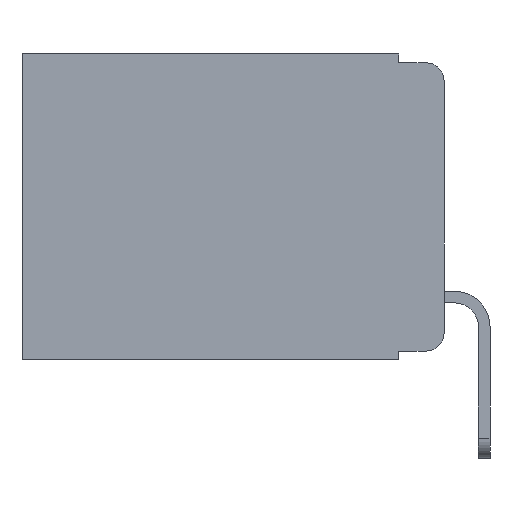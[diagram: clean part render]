
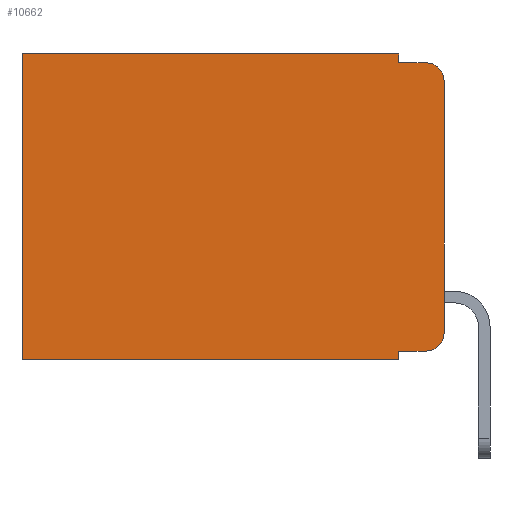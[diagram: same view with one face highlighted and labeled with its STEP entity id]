
A CAD part, left-side view. The second image highlights one B-rep face of the part: STEP entity #10662.
In plain terms, the highlighted planar face has unit normal (-1, 0, 0).
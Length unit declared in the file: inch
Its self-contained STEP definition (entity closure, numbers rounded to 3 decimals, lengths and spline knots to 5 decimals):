
#500 = FACE_OUTER_BOUND ( 'NONE', #8972, .T. ) ;
#1177 = CARTESIAN_POINT ( 'NONE',  ( 0.298, 0.051, 0. ) ) ;
#1775 = CARTESIAN_POINT ( 'NONE',  ( 0.298, 0.473, 0. ) ) ;
#1966 = VECTOR ( 'NONE', #8646, 39.37008 ) ;
#2136 = AXIS2_PLACEMENT_3D ( 'NONE', #11107, #2188, #13180 ) ;
#2175 = LINE ( 'NONE', #10441, #15450 ) ;
#2188 = DIRECTION ( 'NONE',  ( -1., 0., 0. ) ) ;
#2218 = ORIENTED_EDGE ( 'NONE', *, *, #2560, .F. ) ;
#2294 = EDGE_CURVE ( 'NONE', #3955, #2691, #2865, .T. ) ;
#2340 = VECTOR ( 'NONE', #8804, 39.37008 ) ;
#2560 = EDGE_CURVE ( 'NONE', #14445, #5333, #2175, .T. ) ;
#2691 = VERTEX_POINT ( 'NONE', #1775 ) ;
#2821 = CARTESIAN_POINT ( 'NONE',  ( 0.298, 0., 0. ) ) ;
#2848 = DIRECTION ( 'NONE',  ( 0., 1., 0. ) ) ;
#2865 = LINE ( 'NONE', #5798, #1966 ) ;
#2953 = VERTEX_POINT ( 'NONE', #11957 ) ;
#3133 = ORIENTED_EDGE ( 'NONE', *, *, #11868, .F. ) ;
#3510 = VERTEX_POINT ( 'NONE', #8682 ) ;
#3591 = ORIENTED_EDGE ( 'NONE', *, *, #7994, .T. ) ;
#3955 = VERTEX_POINT ( 'NONE', #4451 ) ;
#4451 = CARTESIAN_POINT ( 'NONE',  ( 0.298, 0.051, 0. ) ) ;
#5227 = ORIENTED_EDGE ( 'NONE', *, *, #6734, .T. ) ;
#5333 = VERTEX_POINT ( 'NONE', #7651 ) ;
#5467 = ORIENTED_EDGE ( 'NONE', *, *, #2294, .T. ) ;
#5698 = CARTESIAN_POINT ( 'NONE',  ( 0.298, 0.473, 0. ) ) ;
#5716 = CARTESIAN_POINT ( 'NONE',  ( 0.298, 0.051, -0.343 ) ) ;
#5798 = CARTESIAN_POINT ( 'NONE',  ( 0.298, 0., 0. ) ) ;
#5954 = VERTEX_POINT ( 'NONE', #15307 ) ;
#6241 = LINE ( 'NONE', #5698, #2340 ) ;
#6310 = CARTESIAN_POINT ( 'NONE',  ( 0.298, 0., -0.03 ) ) ;
#6734 = EDGE_CURVE ( 'NONE', #14445, #11534, #11903, .T. ) ;
#6886 = VECTOR ( 'NONE', #10620, 39.37008 ) ;
#6890 = VERTEX_POINT ( 'NONE', #8103 ) ;
#7211 = DIRECTION ( 'NONE',  ( 0., 0., -1. ) ) ;
#7340 = EDGE_CURVE ( 'NONE', #6890, #11534, #14330, .T. ) ;
#7443 = ORIENTED_EDGE ( 'NONE', *, *, #7914, .F. ) ;
#7535 = EDGE_CURVE ( 'NONE', #3955, #6890, #14315, .T. ) ;
#7651 = CARTESIAN_POINT ( 'NONE',  ( 0.298, 0., -0.313 ) ) ;
#7773 = VERTEX_POINT ( 'NONE', #5716 ) ;
#7779 = EDGE_CURVE ( 'NONE', #2691, #5954, #6241, .T. ) ;
#7889 = VECTOR ( 'NONE', #16439, 39.37008 ) ;
#7914 = EDGE_CURVE ( 'NONE', #2953, #7773, #16434, .T. ) ;
#7994 = EDGE_CURVE ( 'NONE', #2953, #3510, #12481, .T. ) ;
#8088 = ORIENTED_EDGE ( 'NONE', *, *, #7340, .F. ) ;
#8102 = ORIENTED_EDGE ( 'NONE', *, *, #8116, .T. ) ;
#8103 = CARTESIAN_POINT ( 'NONE',  ( 0.298, 0.051, -0.01 ) ) ;
#8116 = EDGE_CURVE ( 'NONE', #3510, #5333, #12986, .T. ) ;
#8257 = VECTOR ( 'NONE', #2848, 39.37008 ) ;
#8520 = PLANE ( 'NONE',  #10158 ) ;
#8646 = DIRECTION ( 'NONE',  ( 0., 1., 0. ) ) ;
#8682 = CARTESIAN_POINT ( 'NONE',  ( 0.298, 0.02, -0.333 ) ) ;
#8804 = DIRECTION ( 'NONE',  ( 0., 0., -1. ) ) ;
#8972 = EDGE_LOOP ( 'NONE', ( #2218, #5227, #8088, #15824, #5467, #9133, #3133, #7443, #3591, #8102 ) ) ;
#9133 = ORIENTED_EDGE ( 'NONE', *, *, #7779, .T. ) ;
#10158 = AXIS2_PLACEMENT_3D ( 'NONE', #2821, #14542, #7211 ) ;
#10441 = CARTESIAN_POINT ( 'NONE',  ( 0.298, 0., 0. ) ) ;
#10450 = DIRECTION ( 'NONE',  ( 0., -1., 0. ) ) ;
#10620 = DIRECTION ( 'NONE',  ( 0., 0., -1. ) ) ;
#10647 = AXIS2_PLACEMENT_3D ( 'NONE', #13116, #11872, #11854 ) ;
#10662 = ADVANCED_FACE ( 'NONE', ( #500 ), #8520, .F. ) ;
#11107 = CARTESIAN_POINT ( 'NONE',  ( 0.298, 0.02, -0.03 ) ) ;
#11154 = CARTESIAN_POINT ( 'NONE',  ( 0.298, 0., -0.343 ) ) ;
#11534 = VERTEX_POINT ( 'NONE', #15153 ) ;
#11631 = CARTESIAN_POINT ( 'NONE',  ( 0.298, 0.051, 0. ) ) ;
#11662 = LINE ( 'NONE', #11154, #8257 ) ;
#11854 = DIRECTION ( 'NONE',  ( 0., 0., -1. ) ) ;
#11868 = EDGE_CURVE ( 'NONE', #7773, #5954, #11662, .T. ) ;
#11872 = DIRECTION ( 'NONE',  ( -1., 0., 0. ) ) ;
#11903 = CIRCLE ( 'NONE', #2136, 0.02 ) ;
#11957 = CARTESIAN_POINT ( 'NONE',  ( 0.298, 0.051, -0.333 ) ) ;
#12481 = LINE ( 'NONE', #15262, #14749 ) ;
#12986 = CIRCLE ( 'NONE', #10647, 0.02 ) ;
#13116 = CARTESIAN_POINT ( 'NONE',  ( 0.298, 0.02, -0.313 ) ) ;
#13180 = DIRECTION ( 'NONE',  ( 0., 0., -1. ) ) ;
#13746 = DIRECTION ( 'NONE',  ( 0., -1., 0. ) ) ;
#13994 = VECTOR ( 'NONE', #13746, 39.37008 ) ;
#14315 = LINE ( 'NONE', #1177, #7889 ) ;
#14330 = LINE ( 'NONE', #16086, #13994 ) ;
#14445 = VERTEX_POINT ( 'NONE', #6310 ) ;
#14497 = DIRECTION ( 'NONE',  ( 0., 0., -1. ) ) ;
#14542 = DIRECTION ( 'NONE',  ( 1., 0., 0. ) ) ;
#14749 = VECTOR ( 'NONE', #10450, 39.37008 ) ;
#15153 = CARTESIAN_POINT ( 'NONE',  ( 0.298, 0.02, -0.01 ) ) ;
#15262 = CARTESIAN_POINT ( 'NONE',  ( 0.298, 0.051, -0.333 ) ) ;
#15307 = CARTESIAN_POINT ( 'NONE',  ( 0.298, 0.473, -0.343 ) ) ;
#15450 = VECTOR ( 'NONE', #14497, 39.37008 ) ;
#15824 = ORIENTED_EDGE ( 'NONE', *, *, #7535, .F. ) ;
#16086 = CARTESIAN_POINT ( 'NONE',  ( 0.298, 0.051, -0.01 ) ) ;
#16434 = LINE ( 'NONE', #11631, #6886 ) ;
#16439 = DIRECTION ( 'NONE',  ( 0., 0., -1. ) ) ;
